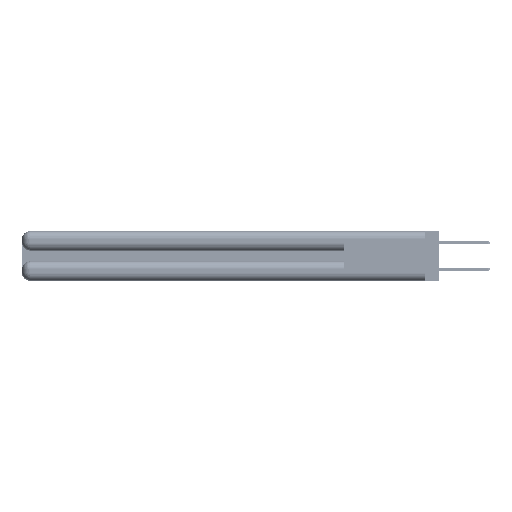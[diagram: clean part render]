
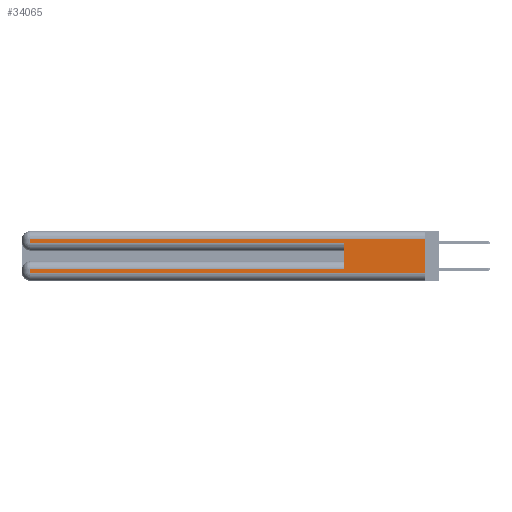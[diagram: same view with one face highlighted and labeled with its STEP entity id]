
A CAD part, left-side view. The second image highlights one B-rep face of the part: STEP entity #34065.
In plain terms, the highlighted planar face has unit normal (-1, 0, 0).
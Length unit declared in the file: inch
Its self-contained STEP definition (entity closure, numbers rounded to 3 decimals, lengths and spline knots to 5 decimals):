
#1082 = ORIENTED_EDGE ( 'NONE', *, *, #33220, .T. ) ;
#1174 = AXIS2_PLACEMENT_3D ( 'NONE', #20655, #49748, #24829 ) ;
#1181 = DIRECTION ( 'NONE',  ( 0., 1., 0. ) ) ;
#2993 = ORIENTED_EDGE ( 'NONE', *, *, #3169, .T. ) ;
#3169 = EDGE_CURVE ( 'NONE', #53315, #51163, #31426, .T. ) ;
#5930 = CARTESIAN_POINT ( 'NONE',  ( 0., 2.94, 0.06 ) ) ;
#7464 = CARTESIAN_POINT ( 'NONE',  ( 0., 2.94, 0.37 ) ) ;
#7507 = EDGE_LOOP ( 'NONE', ( #20005, #2993, #1082, #47986, #49325, #8925, #29208, #12236 ) ) ;
#8482 = VECTOR ( 'NONE', #16856, 39.37008 ) ;
#8925 = ORIENTED_EDGE ( 'NONE', *, *, #48941, .T. ) ;
#9602 = CARTESIAN_POINT ( 'NONE',  ( 0., 0., 0.37 ) ) ;
#9952 = CARTESIAN_POINT ( 'NONE',  ( 0., 0., 0.06 ) ) ;
#10492 = CARTESIAN_POINT ( 'NONE',  ( 0., 2.94, 0.37 ) ) ;
#12236 = ORIENTED_EDGE ( 'NONE', *, *, #40716, .T. ) ;
#12255 = CARTESIAN_POINT ( 'NONE',  ( 0., 0., 0.31 ) ) ;
#12638 = CARTESIAN_POINT ( 'NONE',  ( 0., 0., 0.285 ) ) ;
#12662 = CARTESIAN_POINT ( 'NONE',  ( 0., 2.94, 0.085 ) ) ;
#13614 = CARTESIAN_POINT ( 'NONE',  ( 0., 0., 0.085 ) ) ;
#14247 = CARTESIAN_POINT ( 'NONE',  ( 0., 0., 0.06 ) ) ;
#14379 = EDGE_CURVE ( 'NONE', #53315, #17049, #35367, .T. ) ;
#14793 = LINE ( 'NONE', #29601, #33035 ) ;
#16756 = EDGE_CURVE ( 'NONE', #53657, #32908, #40382, .T. ) ;
#16856 = DIRECTION ( 'NONE',  ( 0., -1., 0. ) ) ;
#17049 = VERTEX_POINT ( 'NONE', #14247 ) ;
#17244 = EDGE_CURVE ( 'NONE', #53653, #50289, #47478, .T. ) ;
#18879 = DIRECTION ( 'NONE',  ( 0., 1., 0. ) ) ;
#18887 = DIRECTION ( 'NONE',  ( 0., 0., -1. ) ) ;
#20005 = ORIENTED_EDGE ( 'NONE', *, *, #14379, .F. ) ;
#20655 = CARTESIAN_POINT ( 'NONE',  ( 0., 0., 0.37 ) ) ;
#21062 = CARTESIAN_POINT ( 'NONE',  ( 0., 2.94, 0.285 ) ) ;
#21229 = DIRECTION ( 'NONE',  ( 0., 0., 1. ) ) ;
#24339 = VECTOR ( 'NONE', #42890, 39.37008 ) ;
#24829 = DIRECTION ( 'NONE',  ( 0., 0., -1. ) ) ;
#25318 = CARTESIAN_POINT ( 'NONE',  ( 0., 0.6, 0.285 ) ) ;
#29208 = ORIENTED_EDGE ( 'NONE', *, *, #17244, .T. ) ;
#29601 = CARTESIAN_POINT ( 'NONE',  ( 0., 0.6, 0.145 ) ) ;
#31426 = LINE ( 'NONE', #43406, #39821 ) ;
#32908 = VERTEX_POINT ( 'NONE', #25318 ) ;
#33035 = VECTOR ( 'NONE', #21229, 39.37008 ) ;
#33220 = EDGE_CURVE ( 'NONE', #51163, #53657, #48893, .T. ) ;
#34065 = ADVANCED_FACE ( 'NONE', ( #40296 ), #45535, .F. ) ;
#34233 = VECTOR ( 'NONE', #1181, 39.37008 ) ;
#35367 = LINE ( 'NONE', #9602, #24339 ) ;
#36498 = VECTOR ( 'NONE', #18887, 39.37008 ) ;
#38158 = EDGE_CURVE ( 'NONE', #40389, #32908, #14793, .T. ) ;
#38888 = DIRECTION ( 'NONE',  ( 0., -1., 0. ) ) ;
#39821 = VECTOR ( 'NONE', #18879, 39.37008 ) ;
#40296 = FACE_OUTER_BOUND ( 'NONE', #7507, .T. ) ;
#40382 = LINE ( 'NONE', #12638, #8482 ) ;
#40389 = VERTEX_POINT ( 'NONE', #49700 ) ;
#40716 = EDGE_CURVE ( 'NONE', #50289, #17049, #43096, .T. ) ;
#42890 = DIRECTION ( 'NONE',  ( 0., 0., -1. ) ) ;
#43096 = LINE ( 'NONE', #9952, #52894 ) ;
#43406 = CARTESIAN_POINT ( 'NONE',  ( 0., 0., 0.31 ) ) ;
#44074 = CARTESIAN_POINT ( 'NONE',  ( 0., 2.94, 0.31 ) ) ;
#44953 = DIRECTION ( 'NONE',  ( 0., 0., -1. ) ) ;
#45304 = LINE ( 'NONE', #13614, #34233 ) ;
#45535 = PLANE ( 'NONE',  #1174 ) ;
#46188 = VECTOR ( 'NONE', #44953, 39.37008 ) ;
#47478 = LINE ( 'NONE', #7464, #46188 ) ;
#47986 = ORIENTED_EDGE ( 'NONE', *, *, #16756, .T. ) ;
#48893 = LINE ( 'NONE', #10492, #36498 ) ;
#48941 = EDGE_CURVE ( 'NONE', #40389, #53653, #45304, .T. ) ;
#49325 = ORIENTED_EDGE ( 'NONE', *, *, #38158, .F. ) ;
#49700 = CARTESIAN_POINT ( 'NONE',  ( 0., 0.6, 0.085 ) ) ;
#49748 = DIRECTION ( 'NONE',  ( 1., 0., 0. ) ) ;
#50289 = VERTEX_POINT ( 'NONE', #5930 ) ;
#51163 = VERTEX_POINT ( 'NONE', #44074 ) ;
#52894 = VECTOR ( 'NONE', #38888, 39.37008 ) ;
#53315 = VERTEX_POINT ( 'NONE', #12255 ) ;
#53653 = VERTEX_POINT ( 'NONE', #12662 ) ;
#53657 = VERTEX_POINT ( 'NONE', #21062 ) ;
